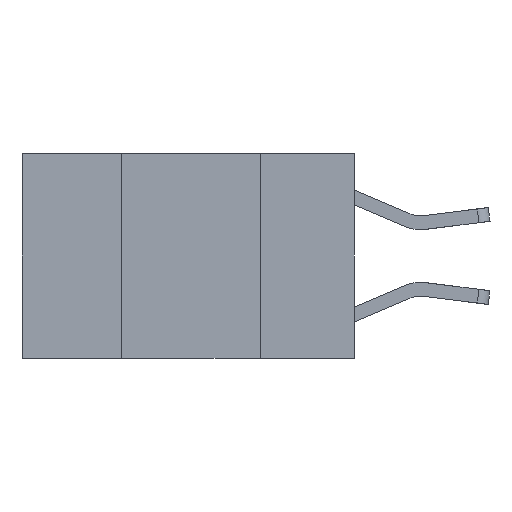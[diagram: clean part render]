
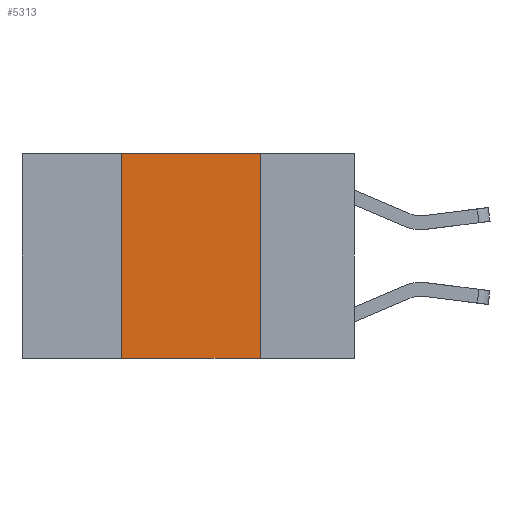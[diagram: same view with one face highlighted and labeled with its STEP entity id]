
A CAD part, left-side view. The second image highlights one B-rep face of the part: STEP entity #5313.
In plain terms, the highlighted planar face has unit normal (-1, 0, 0).
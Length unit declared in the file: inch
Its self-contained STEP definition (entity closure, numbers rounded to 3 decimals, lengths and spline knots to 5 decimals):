
#174 = CARTESIAN_POINT ( 'NONE',  ( 0., 0.42, 0. ) ) ;
#400 = DIRECTION ( 'NONE',  ( 0., 0., -1. ) ) ;
#721 = LINE ( 'NONE', #2685, #5608 ) ;
#1080 = CARTESIAN_POINT ( 'NONE',  ( 0., 0.6, 0. ) ) ;
#1094 = LINE ( 'NONE', #1695, #4456 ) ;
#1170 = VECTOR ( 'NONE', #6761, 39.37008 ) ;
#1676 = CARTESIAN_POINT ( 'NONE',  ( 0., 0.42, -0.37 ) ) ;
#1695 = CARTESIAN_POINT ( 'NONE',  ( 0., 0.42, 0. ) ) ;
#1836 = DIRECTION ( 'NONE',  ( 0., -1., 0. ) ) ;
#1966 = LINE ( 'NONE', #4035, #1170 ) ;
#2299 = FACE_OUTER_BOUND ( 'NONE', #8521, .T. ) ;
#2685 = CARTESIAN_POINT ( 'NONE',  ( 0., 0.6, 0. ) ) ;
#3342 = ORIENTED_EDGE ( 'NONE', *, *, #4490, .T. ) ;
#3372 = VERTEX_POINT ( 'NONE', #4630 ) ;
#3468 = VERTEX_POINT ( 'NONE', #174 ) ;
#3830 = VERTEX_POINT ( 'NONE', #1676 ) ;
#3987 = ORIENTED_EDGE ( 'NONE', *, *, #5916, .F. ) ;
#4035 = CARTESIAN_POINT ( 'NONE',  ( 0., 0.17, 0. ) ) ;
#4456 = VECTOR ( 'NONE', #7204, 39.37008 ) ;
#4490 = EDGE_CURVE ( 'NONE', #3830, #6727, #7944, .T. ) ;
#4630 = CARTESIAN_POINT ( 'NONE',  ( 0., 0.17, 0. ) ) ;
#5313 = ADVANCED_FACE ( 'NONE', ( #2299 ), #7743, .F. ) ;
#5608 = VECTOR ( 'NONE', #8692, 39.37008 ) ;
#5795 = VECTOR ( 'NONE', #1836, 39.37008 ) ;
#5813 = CARTESIAN_POINT ( 'NONE',  ( 0., 0.17, -0.37 ) ) ;
#5916 = EDGE_CURVE ( 'NONE', #3830, #3468, #1094, .T. ) ;
#5994 = EDGE_CURVE ( 'NONE', #3468, #3372, #721, .T. ) ;
#6086 = EDGE_CURVE ( 'NONE', #3372, #6727, #1966, .T. ) ;
#6727 = VERTEX_POINT ( 'NONE', #5813 ) ;
#6761 = DIRECTION ( 'NONE',  ( 0., 0., -1. ) ) ;
#7198 = ORIENTED_EDGE ( 'NONE', *, *, #5994, .F. ) ;
#7204 = DIRECTION ( 'NONE',  ( 0., 0., 1. ) ) ;
#7234 = DIRECTION ( 'NONE',  ( 1., 0., 0. ) ) ;
#7713 = ORIENTED_EDGE ( 'NONE', *, *, #6086, .F. ) ;
#7743 = PLANE ( 'NONE',  #7750 ) ;
#7750 = AXIS2_PLACEMENT_3D ( 'NONE', #1080, #7234, #400 ) ;
#7944 = LINE ( 'NONE', #8035, #5795 ) ;
#8035 = CARTESIAN_POINT ( 'NONE',  ( 0., 0.6, -0.37 ) ) ;
#8521 = EDGE_LOOP ( 'NONE', ( #7713, #7198, #3987, #3342 ) ) ;
#8692 = DIRECTION ( 'NONE',  ( 0., -1., 0. ) ) ;
